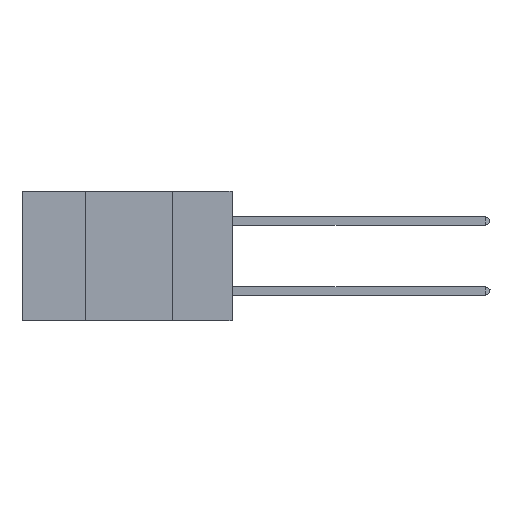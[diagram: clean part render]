
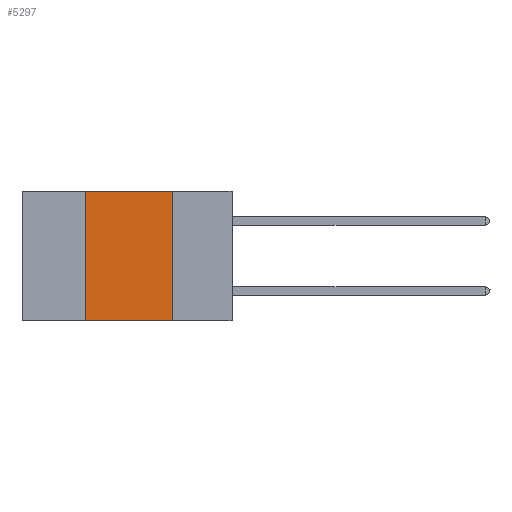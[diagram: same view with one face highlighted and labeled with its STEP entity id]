
A CAD part, left-side view. The second image highlights one B-rep face of the part: STEP entity #5297.
In plain terms, the highlighted planar face has unit normal (-1, 0, 0).
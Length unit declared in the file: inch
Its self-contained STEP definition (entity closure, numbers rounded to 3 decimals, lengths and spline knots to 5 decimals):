
#1671 = EDGE_CURVE ( 'NONE', #18486, #14056, #36211, .T. ) ;
#4244 = VERTEX_POINT ( 'NONE', #34947 ) ;
#5297 = ADVANCED_FACE ( 'NONE', ( #11343 ), #16948, .F. ) ;
#5578 = AXIS2_PLACEMENT_3D ( 'NONE', #8116, #23835, #13925 ) ;
#6658 = CARTESIAN_POINT ( 'NONE',  ( 0., 0.6, -0.37 ) ) ;
#8116 = CARTESIAN_POINT ( 'NONE',  ( 0., 0.6, 0. ) ) ;
#9749 = EDGE_CURVE ( 'NONE', #37453, #4244, #24860, .T. ) ;
#10889 = CARTESIAN_POINT ( 'NONE',  ( 0., 0.42, -0.37 ) ) ;
#10941 = EDGE_CURVE ( 'NONE', #37453, #18486, #16909, .T. ) ;
#11343 = FACE_OUTER_BOUND ( 'NONE', #26669, .T. ) ;
#12120 = CARTESIAN_POINT ( 'NONE',  ( 0., 0.17, 0. ) ) ;
#13329 = CARTESIAN_POINT ( 'NONE',  ( 0., 0.42, 0. ) ) ;
#13925 = DIRECTION ( 'NONE',  ( 0., 0., -1. ) ) ;
#14056 = VERTEX_POINT ( 'NONE', #27052 ) ;
#14749 = DIRECTION ( 'NONE',  ( 0., -1., 0. ) ) ;
#16486 = VECTOR ( 'NONE', #21613, 39.37008 ) ;
#16909 = LINE ( 'NONE', #13329, #34135 ) ;
#16948 = PLANE ( 'NONE',  #5578 ) ;
#18486 = VERTEX_POINT ( 'NONE', #23134 ) ;
#21613 = DIRECTION ( 'NONE',  ( 0., 0., -1. ) ) ;
#23134 = CARTESIAN_POINT ( 'NONE',  ( 0., 0.42, 0. ) ) ;
#23835 = DIRECTION ( 'NONE',  ( 1., 0., 0. ) ) ;
#24658 = ORIENTED_EDGE ( 'NONE', *, *, #9749, .T. ) ;
#24842 = LINE ( 'NONE', #12120, #16486 ) ;
#24860 = LINE ( 'NONE', #6658, #27337 ) ;
#26669 = EDGE_LOOP ( 'NONE', ( #27976, #30491, #39758, #24658 ) ) ;
#27052 = CARTESIAN_POINT ( 'NONE',  ( 0., 0.17, 0. ) ) ;
#27337 = VECTOR ( 'NONE', #35010, 39.37008 ) ;
#27976 = ORIENTED_EDGE ( 'NONE', *, *, #28449, .F. ) ;
#28449 = EDGE_CURVE ( 'NONE', #14056, #4244, #24842, .T. ) ;
#30491 = ORIENTED_EDGE ( 'NONE', *, *, #1671, .F. ) ;
#33594 = CARTESIAN_POINT ( 'NONE',  ( 0., 0.6, 0. ) ) ;
#34135 = VECTOR ( 'NONE', #39415, 39.37008 ) ;
#34947 = CARTESIAN_POINT ( 'NONE',  ( 0., 0.17, -0.37 ) ) ;
#35010 = DIRECTION ( 'NONE',  ( 0., -1., 0. ) ) ;
#36211 = LINE ( 'NONE', #33594, #38161 ) ;
#37453 = VERTEX_POINT ( 'NONE', #10889 ) ;
#38161 = VECTOR ( 'NONE', #14749, 39.37008 ) ;
#39415 = DIRECTION ( 'NONE',  ( 0., 0., 1. ) ) ;
#39758 = ORIENTED_EDGE ( 'NONE', *, *, #10941, .F. ) ;
